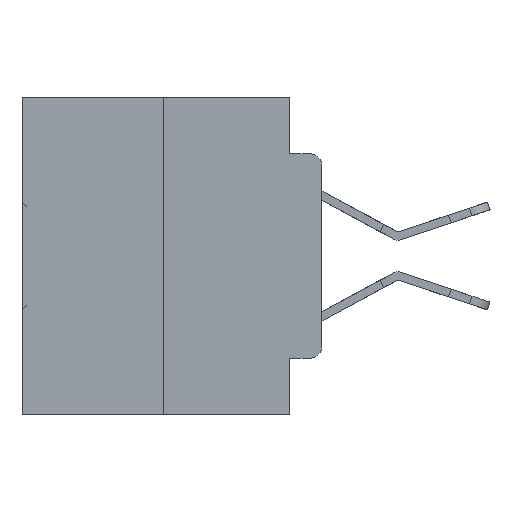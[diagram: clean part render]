
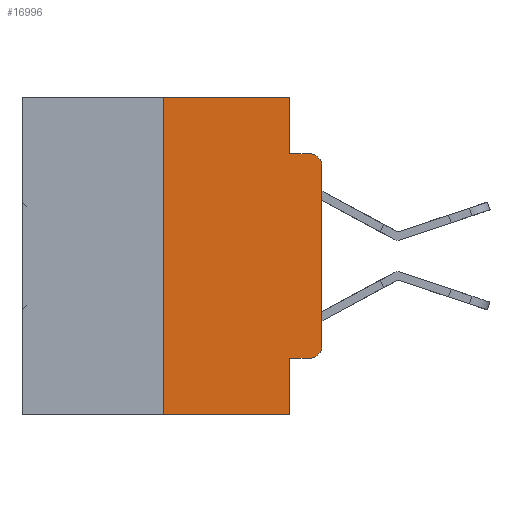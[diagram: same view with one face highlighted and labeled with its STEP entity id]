
A CAD part, left-side view. The second image highlights one B-rep face of the part: STEP entity #16996.
In plain terms, the highlighted planar face has unit normal (-1, 0, 0).
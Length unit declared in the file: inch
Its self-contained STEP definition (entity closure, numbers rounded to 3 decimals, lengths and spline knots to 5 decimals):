
#1300 = VERTEX_POINT ( 'NONE', #34910 ) ;
#1913 = VERTEX_POINT ( 'NONE', #30912 ) ;
#2635 = ORIENTED_EDGE ( 'NONE', *, *, #32192, .F. ) ;
#3679 = ORIENTED_EDGE ( 'NONE', *, *, #17718, .F. ) ;
#3786 = VECTOR ( 'NONE', #6636, 39.37008 ) ;
#4101 = VERTEX_POINT ( 'NONE', #31019 ) ;
#4341 = DIRECTION ( 'NONE',  ( 0., 0., -1. ) ) ;
#4374 = EDGE_LOOP ( 'NONE', ( #12500, #13254, #11292, #3679, #33942, #2635, #23787, #35383, #20045, #31250 ) ) ;
#5256 = AXIS2_PLACEMENT_3D ( 'NONE', #32105, #15891, #9986 ) ;
#6317 = VECTOR ( 'NONE', #29275, 39.37008 ) ;
#6601 = VERTEX_POINT ( 'NONE', #14346 ) ;
#6636 = DIRECTION ( 'NONE',  ( 0., -1., 0. ) ) ;
#7551 = LINE ( 'NONE', #10448, #8413 ) ;
#8355 = VERTEX_POINT ( 'NONE', #28059 ) ;
#8413 = VECTOR ( 'NONE', #15650, 39.37008 ) ;
#9093 = EDGE_CURVE ( 'NONE', #1300, #16905, #16969, .T. ) ;
#9779 = LINE ( 'NONE', #26239, #19993 ) ;
#9948 = DIRECTION ( 'NONE',  ( 0., -1., 0. ) ) ;
#9986 = DIRECTION ( 'NONE',  ( 0., 0., -1. ) ) ;
#10425 = VERTEX_POINT ( 'NONE', #10952 ) ;
#10448 = CARTESIAN_POINT ( 'NONE',  ( 0., 0.051, -0.0885 ) ) ;
#10952 = CARTESIAN_POINT ( 'NONE',  ( 0., 0.02, -0.0885 ) ) ;
#11292 = ORIENTED_EDGE ( 'NONE', *, *, #12876, .F. ) ;
#11541 = CARTESIAN_POINT ( 'NONE',  ( 0., 0.051, -0.4115 ) ) ;
#12500 = ORIENTED_EDGE ( 'NONE', *, *, #19182, .T. ) ;
#12876 = EDGE_CURVE ( 'NONE', #6601, #10425, #7551, .T. ) ;
#13082 = EDGE_CURVE ( 'NONE', #4101, #1300, #25325, .T. ) ;
#13254 = ORIENTED_EDGE ( 'NONE', *, *, #19981, .T. ) ;
#14346 = CARTESIAN_POINT ( 'NONE',  ( 0., 0.051, -0.0885 ) ) ;
#15220 = AXIS2_PLACEMENT_3D ( 'NONE', #16638, #16817, #16453 ) ;
#15619 = EDGE_CURVE ( 'NONE', #4101, #29472, #34437, .T. ) ;
#15650 = DIRECTION ( 'NONE',  ( 0., -1., 0. ) ) ;
#15891 = DIRECTION ( 'NONE',  ( -1., 0., 0. ) ) ;
#15945 = CARTESIAN_POINT ( 'NONE',  ( 0., 0.25, 0. ) ) ;
#15971 = LINE ( 'NONE', #18304, #6317 ) ;
#16156 = VECTOR ( 'NONE', #35206, 39.37008 ) ;
#16214 = EDGE_CURVE ( 'NONE', #27443, #29472, #30540, .T. ) ;
#16453 = DIRECTION ( 'NONE',  ( 0., 0., -1. ) ) ;
#16638 = CARTESIAN_POINT ( 'NONE',  ( 0., 0.02, -0.3915 ) ) ;
#16706 = LINE ( 'NONE', #29677, #26441 ) ;
#16817 = DIRECTION ( 'NONE',  ( -1., 0., 0. ) ) ;
#16905 = VERTEX_POINT ( 'NONE', #27324 ) ;
#16969 = CIRCLE ( 'NONE', #15220, 0.02 ) ;
#16996 = ADVANCED_FACE ( 'NONE', ( #30491 ), #30307, .F. ) ;
#17718 = EDGE_CURVE ( 'NONE', #8355, #6601, #15971, .T. ) ;
#18304 = CARTESIAN_POINT ( 'NONE',  ( 0., 0.051, 0. ) ) ;
#18907 = CARTESIAN_POINT ( 'NONE',  ( 0., 0.25, -0.5 ) ) ;
#19182 = EDGE_CURVE ( 'NONE', #16905, #1913, #16706, .T. ) ;
#19981 = EDGE_CURVE ( 'NONE', #1913, #10425, #28820, .T. ) ;
#19993 = VECTOR ( 'NONE', #9948, 39.37008 ) ;
#20045 = ORIENTED_EDGE ( 'NONE', *, *, #13082, .T. ) ;
#20726 = CARTESIAN_POINT ( 'NONE',  ( 0., 0.051, 0. ) ) ;
#21566 = DIRECTION ( 'NONE',  ( 0., 0., 1. ) ) ;
#22957 = VECTOR ( 'NONE', #30170, 39.37008 ) ;
#23067 = CARTESIAN_POINT ( 'NONE',  ( 0., 0.25, 0. ) ) ;
#23459 = VECTOR ( 'NONE', #4341, 39.37008 ) ;
#23787 = ORIENTED_EDGE ( 'NONE', *, *, #16214, .T. ) ;
#24507 = DIRECTION ( 'NONE',  ( 1., 0., 0. ) ) ;
#25325 = LINE ( 'NONE', #11541, #3786 ) ;
#25585 = CARTESIAN_POINT ( 'NONE',  ( 0., 0.051, -0.5 ) ) ;
#26239 = CARTESIAN_POINT ( 'NONE',  ( 0., 0.473, 0. ) ) ;
#26441 = VECTOR ( 'NONE', #21566, 39.37008 ) ;
#27324 = CARTESIAN_POINT ( 'NONE',  ( 0., 0., -0.3915 ) ) ;
#27443 = VERTEX_POINT ( 'NONE', #18907 ) ;
#27575 = CARTESIAN_POINT ( 'NONE',  ( 0., 0.473, 0. ) ) ;
#28059 = CARTESIAN_POINT ( 'NONE',  ( 0., 0.051, 0. ) ) ;
#28820 = CIRCLE ( 'NONE', #5256, 0.02 ) ;
#29275 = DIRECTION ( 'NONE',  ( 0., 0., -1. ) ) ;
#29424 = EDGE_CURVE ( 'NONE', #35518, #8355, #9779, .T. ) ;
#29431 = LINE ( 'NONE', #15945, #16156 ) ;
#29472 = VERTEX_POINT ( 'NONE', #25585 ) ;
#29677 = CARTESIAN_POINT ( 'NONE',  ( 0., 0., 0. ) ) ;
#30170 = DIRECTION ( 'NONE',  ( 0., -1., 0. ) ) ;
#30307 = PLANE ( 'NONE',  #32215 ) ;
#30491 = FACE_OUTER_BOUND ( 'NONE', #4374, .T. ) ;
#30540 = LINE ( 'NONE', #32903, #22957 ) ;
#30912 = CARTESIAN_POINT ( 'NONE',  ( 0., 0., -0.1085 ) ) ;
#31019 = CARTESIAN_POINT ( 'NONE',  ( 0., 0.051, -0.4115 ) ) ;
#31250 = ORIENTED_EDGE ( 'NONE', *, *, #9093, .T. ) ;
#32105 = CARTESIAN_POINT ( 'NONE',  ( 0., 0.02, -0.1085 ) ) ;
#32192 = EDGE_CURVE ( 'NONE', #27443, #35518, #29431, .T. ) ;
#32215 = AXIS2_PLACEMENT_3D ( 'NONE', #27575, #24507, #32859 ) ;
#32859 = DIRECTION ( 'NONE',  ( 0., 0., -1. ) ) ;
#32903 = CARTESIAN_POINT ( 'NONE',  ( 0., 0.473, -0.5 ) ) ;
#33942 = ORIENTED_EDGE ( 'NONE', *, *, #29424, .F. ) ;
#34437 = LINE ( 'NONE', #20726, #23459 ) ;
#34910 = CARTESIAN_POINT ( 'NONE',  ( 0., 0.02, -0.4115 ) ) ;
#35206 = DIRECTION ( 'NONE',  ( 0., 0., 1. ) ) ;
#35383 = ORIENTED_EDGE ( 'NONE', *, *, #15619, .F. ) ;
#35518 = VERTEX_POINT ( 'NONE', #23067 ) ;
